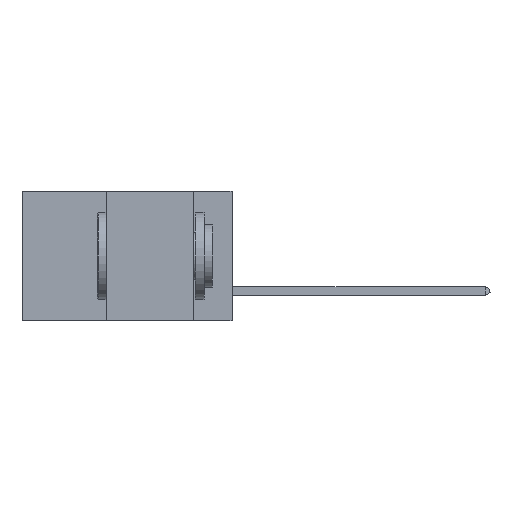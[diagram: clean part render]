
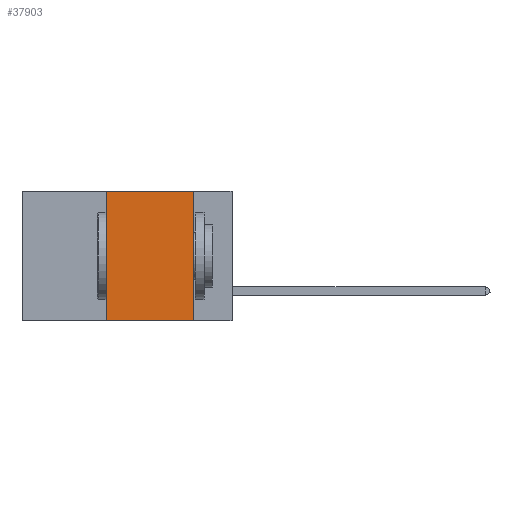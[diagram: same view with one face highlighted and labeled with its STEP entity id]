
A CAD part, left-side view. The second image highlights one B-rep face of the part: STEP entity #37903.
In plain terms, the highlighted planar face has unit normal (-1, 0, 0).
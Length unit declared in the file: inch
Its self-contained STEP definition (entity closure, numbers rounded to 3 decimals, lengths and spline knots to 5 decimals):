
#67 = LINE ( 'NONE', #37676, #17874 ) ;
#203 = CARTESIAN_POINT ( 'NONE',  ( 0., 0.6, 0. ) ) ;
#2084 = PLANE ( 'NONE',  #47799 ) ;
#3527 = VECTOR ( 'NONE', #36153, 39.37008 ) ;
#6057 = CARTESIAN_POINT ( 'NONE',  ( 0., 0.11, 0. ) ) ;
#10148 = CARTESIAN_POINT ( 'NONE',  ( 0., 0.6, 0. ) ) ;
#16218 = LINE ( 'NONE', #203, #49200 ) ;
#16341 = CARTESIAN_POINT ( 'NONE',  ( 0., 0.36, 0. ) ) ;
#17874 = VECTOR ( 'NONE', #29930, 39.37008 ) ;
#21762 = DIRECTION ( 'NONE',  ( 1., 0., 0. ) ) ;
#22036 = VERTEX_POINT ( 'NONE', #48931 ) ;
#22538 = LINE ( 'NONE', #6057, #24375 ) ;
#23513 = ORIENTED_EDGE ( 'NONE', *, *, #49500, .F. ) ;
#24375 = VECTOR ( 'NONE', #33941, 39.37008 ) ;
#25387 = FACE_OUTER_BOUND ( 'NONE', #28058, .T. ) ;
#28058 = EDGE_LOOP ( 'NONE', ( #23513, #43183, #30221, #50146 ) ) ;
#28757 = CARTESIAN_POINT ( 'NONE',  ( 0., 0.11, 0. ) ) ;
#29930 = DIRECTION ( 'NONE',  ( 0., -1., 0. ) ) ;
#30221 = ORIENTED_EDGE ( 'NONE', *, *, #36285, .F. ) ;
#32894 = LINE ( 'NONE', #16341, #3527 ) ;
#33941 = DIRECTION ( 'NONE',  ( 0., 0., -1. ) ) ;
#36153 = DIRECTION ( 'NONE',  ( 0., 0., 1. ) ) ;
#36285 = EDGE_CURVE ( 'NONE', #22036, #42796, #32894, .T. ) ;
#37676 = CARTESIAN_POINT ( 'NONE',  ( 0., 0.6, -0.37 ) ) ;
#37903 = ADVANCED_FACE ( 'NONE', ( #25387 ), #2084, .F. ) ;
#39527 = CARTESIAN_POINT ( 'NONE',  ( 0., 0.36, 0. ) ) ;
#39582 = DIRECTION ( 'NONE',  ( 0., -1., 0. ) ) ;
#39684 = EDGE_CURVE ( 'NONE', #42796, #39817, #16218, .T. ) ;
#39817 = VERTEX_POINT ( 'NONE', #28757 ) ;
#40664 = VERTEX_POINT ( 'NONE', #40867 ) ;
#40867 = CARTESIAN_POINT ( 'NONE',  ( 0., 0.11, -0.37 ) ) ;
#41109 = DIRECTION ( 'NONE',  ( 0., 0., -1. ) ) ;
#41112 = EDGE_CURVE ( 'NONE', #22036, #40664, #67, .T. ) ;
#42796 = VERTEX_POINT ( 'NONE', #39527 ) ;
#43183 = ORIENTED_EDGE ( 'NONE', *, *, #39684, .F. ) ;
#47799 = AXIS2_PLACEMENT_3D ( 'NONE', #10148, #21762, #41109 ) ;
#48931 = CARTESIAN_POINT ( 'NONE',  ( 0., 0.36, -0.37 ) ) ;
#49200 = VECTOR ( 'NONE', #39582, 39.37008 ) ;
#49500 = EDGE_CURVE ( 'NONE', #39817, #40664, #22538, .T. ) ;
#50146 = ORIENTED_EDGE ( 'NONE', *, *, #41112, .T. ) ;
